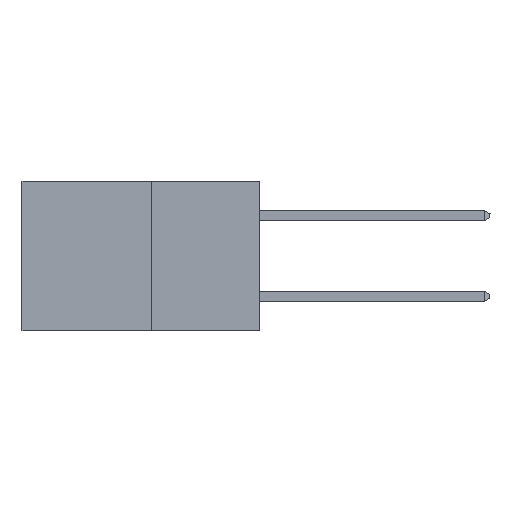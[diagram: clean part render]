
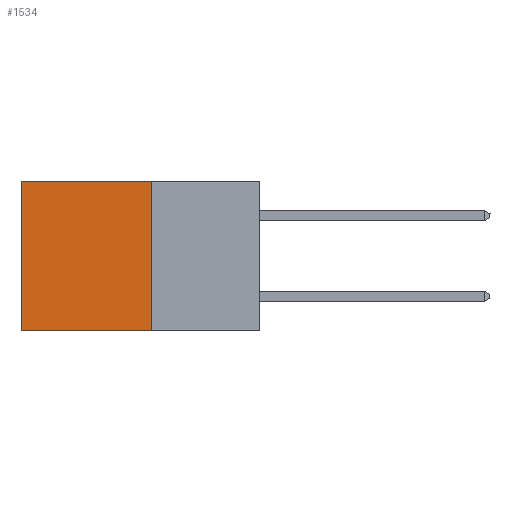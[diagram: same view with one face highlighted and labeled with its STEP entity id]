
A CAD part, left-side view. The second image highlights one B-rep face of the part: STEP entity #1534.
In plain terms, the highlighted planar face has unit normal (-1, 0, 0).
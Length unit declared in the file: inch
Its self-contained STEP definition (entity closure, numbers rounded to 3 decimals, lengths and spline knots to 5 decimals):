
#136 = DIRECTION ( 'NONE',  ( 1., 0., 0. ) ) ;
#165 = DIRECTION ( 'NONE',  ( 0., 0., -1. ) ) ;
#357 = ORIENTED_EDGE ( 'NONE', *, *, #475, .T. ) ;
#392 = CARTESIAN_POINT ( 'NONE',  ( 0.277, 0.27, 0. ) ) ;
#475 = EDGE_CURVE ( 'NONE', #2464, #6938, #7313, .T. ) ;
#622 = EDGE_CURVE ( 'NONE', #6210, #7331, #4829, .T. ) ;
#1130 = FACE_OUTER_BOUND ( 'NONE', #3700, .T. ) ;
#1406 = CARTESIAN_POINT ( 'NONE',  ( 0.277, 0.27, -0.37 ) ) ;
#1534 = ADVANCED_FACE ( 'NONE', ( #1130 ), #2290, .F. ) ;
#1976 = EDGE_CURVE ( 'NONE', #6938, #7331, #6569, .T. ) ;
#2073 = CARTESIAN_POINT ( 'NONE',  ( 0.277, 0.59, 0. ) ) ;
#2290 = PLANE ( 'NONE',  #8366 ) ;
#2348 = VECTOR ( 'NONE', #7832, 39.37008 ) ;
#2438 = CARTESIAN_POINT ( 'NONE',  ( 0.277, 0.27, -0.37 ) ) ;
#2456 = ORIENTED_EDGE ( 'NONE', *, *, #1976, .T. ) ;
#2464 = VERTEX_POINT ( 'NONE', #9348 ) ;
#2858 = DIRECTION ( 'NONE',  ( 0., 1., 0. ) ) ;
#2936 = VECTOR ( 'NONE', #8398, 39.37008 ) ;
#3408 = CARTESIAN_POINT ( 'NONE',  ( 0.277, 0.59, -0.37 ) ) ;
#3508 = LINE ( 'NONE', #10428, #5557 ) ;
#3700 = EDGE_LOOP ( 'NONE', ( #2456, #6916, #8875, #357 ) ) ;
#4829 = LINE ( 'NONE', #7631, #6742 ) ;
#5557 = VECTOR ( 'NONE', #10461, 39.37008 ) ;
#6210 = VERTEX_POINT ( 'NONE', #1406 ) ;
#6569 = LINE ( 'NONE', #6637, #2348 ) ;
#6637 = CARTESIAN_POINT ( 'NONE',  ( 0.277, 0.59, -0.37 ) ) ;
#6742 = VECTOR ( 'NONE', #2858, 39.37008 ) ;
#6916 = ORIENTED_EDGE ( 'NONE', *, *, #622, .F. ) ;
#6938 = VERTEX_POINT ( 'NONE', #2073 ) ;
#7313 = LINE ( 'NONE', #392, #2936 ) ;
#7331 = VERTEX_POINT ( 'NONE', #3408 ) ;
#7437 = EDGE_CURVE ( 'NONE', #2464, #6210, #3508, .T. ) ;
#7631 = CARTESIAN_POINT ( 'NONE',  ( 0.277, 0.27, -0.37 ) ) ;
#7832 = DIRECTION ( 'NONE',  ( 0., 0., -1. ) ) ;
#8366 = AXIS2_PLACEMENT_3D ( 'NONE', #2438, #136, #165 ) ;
#8398 = DIRECTION ( 'NONE',  ( 0., 1., 0. ) ) ;
#8875 = ORIENTED_EDGE ( 'NONE', *, *, #7437, .F. ) ;
#9348 = CARTESIAN_POINT ( 'NONE',  ( 0.277, 0.27, 0. ) ) ;
#10428 = CARTESIAN_POINT ( 'NONE',  ( 0.277, 0.27, -0.37 ) ) ;
#10461 = DIRECTION ( 'NONE',  ( 0., 0., -1. ) ) ;
